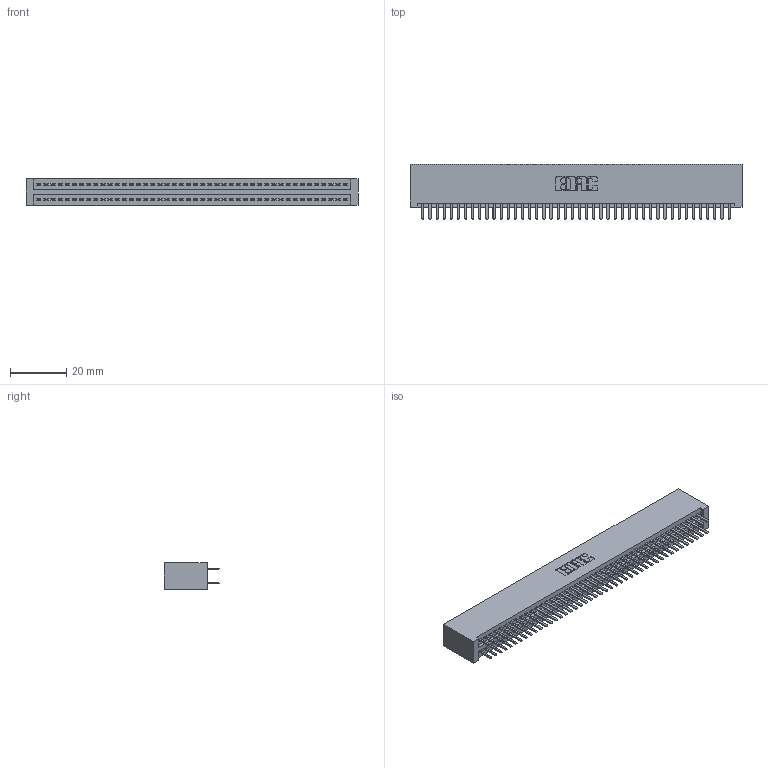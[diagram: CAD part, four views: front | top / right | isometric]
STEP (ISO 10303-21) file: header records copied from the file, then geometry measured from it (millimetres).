
FILE_DESCRIPTION (( 'STEP AP203' ), '1' );
FILE_NAME ('345-088-520-201.STEP', '2019-11-01T10:08:05', ( '' ), ( '' ), 'SwSTEP 2.0', 'SolidWorks 2016', '' );
FILE_SCHEMA (( 'CONFIG_CONTROL_DESIGN' ));
Length unit declared in the file: inch
Products named in the file (3): 345 Part_No Mounting Lugs; 345-088-520-201; 345-292-001_345-293-120
Assembly tree (89 placements, depth 2):
  345-088-520-201
    345 Part_No Mounting Lugs
    345-292-001_345-293-120  x88
Bounding box: 118.36 x 19.68 x 9.4 mm (x, y, z)
Volume: 12093.8 mm3; surface area: 18136.4 mm2
Topology: 89 solids, 89 shells, 4870 faces, 14133 edges, 9186 vertices
Faces by surface type: plane 3156, cylinder 1714
Entity records: 34091 total; most frequent: CARTESIAN_POINT 5724, ORIENTED_EDGE 5646, DIRECTION 5027, EDGE_CURVE 2823, LINE 2519, VECTOR 2519, VERTEX_POINT 1878, AXIS2_PLACEMENT_3D 1254
